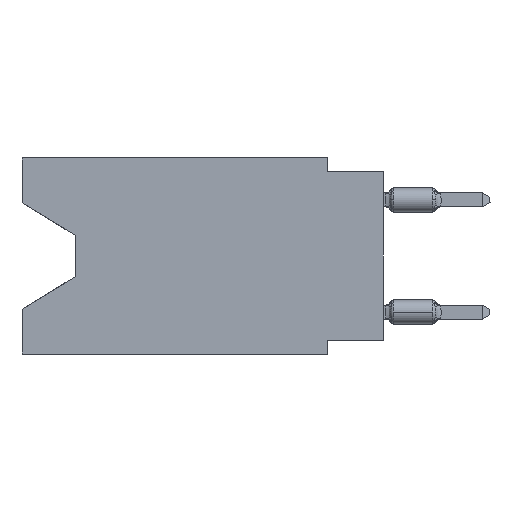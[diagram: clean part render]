
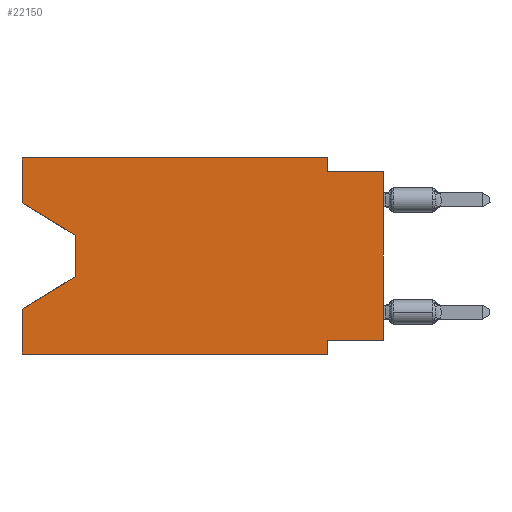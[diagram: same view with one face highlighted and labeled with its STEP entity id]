
A CAD part, left-side view. The second image highlights one B-rep face of the part: STEP entity #22150.
In plain terms, the highlighted planar face has unit normal (-1, 0, 0).
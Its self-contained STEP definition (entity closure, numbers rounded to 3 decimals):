
#695 = EDGE_CURVE ( 'NONE', #2362, #20442, #35936, .T. ) ;
#742 = ORIENTED_EDGE ( 'NONE', *, *, #695, .F. ) ;
#884 = CARTESIAN_POINT ( 'NONE',  ( 0., 2.54, -8.89 ) ) ;
#1107 = ORIENTED_EDGE ( 'NONE', *, *, #3677, .T. ) ;
#2160 = EDGE_CURVE ( 'NONE', #37109, #17321, #24939, .T. ) ;
#2362 = VERTEX_POINT ( 'NONE', #7524 ) ;
#2787 = LINE ( 'NONE', #9051, #23507 ) ;
#3246 = EDGE_CURVE ( 'NONE', #37109, #20442, #7989, .T. ) ;
#3361 = PLANE ( 'NONE',  #5078 ) ;
#3614 = ORIENTED_EDGE ( 'NONE', *, *, #4014, .F. ) ;
#3677 = EDGE_CURVE ( 'NONE', #33360, #17321, #18192, .T. ) ;
#3749 = VERTEX_POINT ( 'NONE', #21628 ) ;
#3898 = CARTESIAN_POINT ( 'NONE',  ( 0., 2.54, 0. ) ) ;
#4014 = EDGE_CURVE ( 'NONE', #3749, #2362, #29357, .T. ) ;
#4444 = CARTESIAN_POINT ( 'NONE',  ( 0., 13.97, -3.505 ) ) ;
#4572 = VECTOR ( 'NONE', #15343, 1000. ) ;
#4796 = VERTEX_POINT ( 'NONE', #14035 ) ;
#4807 = VECTOR ( 'NONE', #16048, 1000. ) ;
#5078 = AXIS2_PLACEMENT_3D ( 'NONE', #14781, #34986, #37645 ) ;
#5910 = VECTOR ( 'NONE', #32430, 1000. ) ;
#7524 = CARTESIAN_POINT ( 'NONE',  ( 0., 2.54, -8.255 ) ) ;
#7536 = VECTOR ( 'NONE', #30665, 1000. ) ;
#7640 = VERTEX_POINT ( 'NONE', #3898 ) ;
#7989 = LINE ( 'NONE', #16561, #25231 ) ;
#8374 = CARTESIAN_POINT ( 'NONE',  ( 0., 0., -0.635 ) ) ;
#8449 = DIRECTION ( 'NONE',  ( 0., -1., 0. ) ) ;
#9051 = CARTESIAN_POINT ( 'NONE',  ( 0., 16.383, -2.038 ) ) ;
#9311 = VECTOR ( 'NONE', #8449, 1000. ) ;
#9855 = CARTESIAN_POINT ( 'NONE',  ( 0., 16.383, -2.038 ) ) ;
#10365 = EDGE_CURVE ( 'NONE', #25892, #14541, #2787, .T. ) ;
#11093 = CARTESIAN_POINT ( 'NONE',  ( 0., 13.97, -5.385 ) ) ;
#11110 = EDGE_CURVE ( 'NONE', #7640, #4796, #14719, .T. ) ;
#11155 = ORIENTED_EDGE ( 'NONE', *, *, #30360, .F. ) ;
#13322 = EDGE_CURVE ( 'NONE', #14541, #33360, #30529, .T. ) ;
#13342 = LINE ( 'NONE', #8374, #29236 ) ;
#13706 = CARTESIAN_POINT ( 'NONE',  ( 0., 2.54, -8.89 ) ) ;
#13920 = ORIENTED_EDGE ( 'NONE', *, *, #31733, .F. ) ;
#14035 = CARTESIAN_POINT ( 'NONE',  ( 0., 2.54, -0.635 ) ) ;
#14541 = VERTEX_POINT ( 'NONE', #19688 ) ;
#14719 = LINE ( 'NONE', #35677, #5910 ) ;
#14781 = CARTESIAN_POINT ( 'NONE',  ( 0., 16.383, 0. ) ) ;
#15343 = DIRECTION ( 'NONE',  ( 0., 0.855, -0.519 ) ) ;
#15907 = CARTESIAN_POINT ( 'NONE',  ( 0., 0., 0. ) ) ;
#16048 = DIRECTION ( 'NONE',  ( 0., 0., -1. ) ) ;
#16106 = VERTEX_POINT ( 'NONE', #26602 ) ;
#16145 = VECTOR ( 'NONE', #23039, 1000. ) ;
#16365 = DIRECTION ( 'NONE',  ( 0., -1., 0. ) ) ;
#16457 = VERTEX_POINT ( 'NONE', #28482 ) ;
#16561 = CARTESIAN_POINT ( 'NONE',  ( 0., 16.383, -8.89 ) ) ;
#16846 = LINE ( 'NONE', #36685, #9311 ) ;
#17127 = VECTOR ( 'NONE', #21240, 1000. ) ;
#17133 = CARTESIAN_POINT ( 'NONE',  ( 0., 16.383, 0. ) ) ;
#17321 = VERTEX_POINT ( 'NONE', #28568 ) ;
#17370 = ORIENTED_EDGE ( 'NONE', *, *, #13322, .T. ) ;
#17723 = DIRECTION ( 'NONE',  ( 0., 1., 0. ) ) ;
#17819 = FACE_OUTER_BOUND ( 'NONE', #32344, .T. ) ;
#18192 = LINE ( 'NONE', #32863, #4572 ) ;
#18201 = CARTESIAN_POINT ( 'NONE',  ( 0., 16.383, -8.89 ) ) ;
#19268 = VECTOR ( 'NONE', #27549, 1000. ) ;
#19688 = CARTESIAN_POINT ( 'NONE',  ( 0., 13.97, -3.505 ) ) ;
#19981 = DIRECTION ( 'NONE',  ( 0., -1., 0. ) ) ;
#20442 = VERTEX_POINT ( 'NONE', #13706 ) ;
#21240 = DIRECTION ( 'NONE',  ( 0., 0., 1. ) ) ;
#21628 = CARTESIAN_POINT ( 'NONE',  ( 0., 0., -8.255 ) ) ;
#21822 = LINE ( 'NONE', #15907, #17127 ) ;
#22085 = CARTESIAN_POINT ( 'NONE',  ( 0., 16.383, 0. ) ) ;
#22150 = ADVANCED_FACE ( 'NONE', ( #17819 ), #3361, .F. ) ;
#23039 = DIRECTION ( 'NONE',  ( 0., 0., 1. ) ) ;
#23507 = VECTOR ( 'NONE', #23523, 1000. ) ;
#23523 = DIRECTION ( 'NONE',  ( 0., -0.855, -0.519 ) ) ;
#24042 = VECTOR ( 'NONE', #17723, 1000. ) ;
#24939 = LINE ( 'NONE', #22085, #7536 ) ;
#25033 = ORIENTED_EDGE ( 'NONE', *, *, #10365, .T. ) ;
#25231 = VECTOR ( 'NONE', #16365, 1000. ) ;
#25892 = VERTEX_POINT ( 'NONE', #9855 ) ;
#26602 = CARTESIAN_POINT ( 'NONE',  ( 0., 0., -0.635 ) ) ;
#27549 = DIRECTION ( 'NONE',  ( 0., 0., -1. ) ) ;
#28482 = CARTESIAN_POINT ( 'NONE',  ( 0., 16.383, 0. ) ) ;
#28568 = CARTESIAN_POINT ( 'NONE',  ( 0., 16.383, -6.852 ) ) ;
#29236 = VECTOR ( 'NONE', #19981, 1000. ) ;
#29357 = LINE ( 'NONE', #35082, #24042 ) ;
#29750 = ORIENTED_EDGE ( 'NONE', *, *, #33854, .F. ) ;
#30272 = ORIENTED_EDGE ( 'NONE', *, *, #2160, .F. ) ;
#30360 = EDGE_CURVE ( 'NONE', #25892, #16457, #34479, .T. ) ;
#30529 = LINE ( 'NONE', #4444, #4807 ) ;
#30665 = DIRECTION ( 'NONE',  ( 0., 0., 1. ) ) ;
#31196 = ORIENTED_EDGE ( 'NONE', *, *, #3246, .T. ) ;
#31733 = EDGE_CURVE ( 'NONE', #16457, #7640, #16846, .T. ) ;
#32344 = EDGE_LOOP ( 'NONE', ( #25033, #17370, #1107, #30272, #31196, #742, #3614, #35200, #29750, #36986, #13920, #11155 ) ) ;
#32430 = DIRECTION ( 'NONE',  ( 0., 0., -1. ) ) ;
#32863 = CARTESIAN_POINT ( 'NONE',  ( 0., 13.97, -5.385 ) ) ;
#33360 = VERTEX_POINT ( 'NONE', #11093 ) ;
#33854 = EDGE_CURVE ( 'NONE', #4796, #16106, #13342, .T. ) ;
#34479 = LINE ( 'NONE', #17133, #16145 ) ;
#34986 = DIRECTION ( 'NONE',  ( 1., 0., 0. ) ) ;
#35082 = CARTESIAN_POINT ( 'NONE',  ( 0., 0., -8.255 ) ) ;
#35200 = ORIENTED_EDGE ( 'NONE', *, *, #35986, .T. ) ;
#35677 = CARTESIAN_POINT ( 'NONE',  ( 0., 2.54, 0. ) ) ;
#35936 = LINE ( 'NONE', #884, #19268 ) ;
#35986 = EDGE_CURVE ( 'NONE', #3749, #16106, #21822, .T. ) ;
#36685 = CARTESIAN_POINT ( 'NONE',  ( 0., 16.383, 0. ) ) ;
#36986 = ORIENTED_EDGE ( 'NONE', *, *, #11110, .F. ) ;
#37109 = VERTEX_POINT ( 'NONE', #18201 ) ;
#37645 = DIRECTION ( 'NONE',  ( 0., 0., -1. ) ) ;
